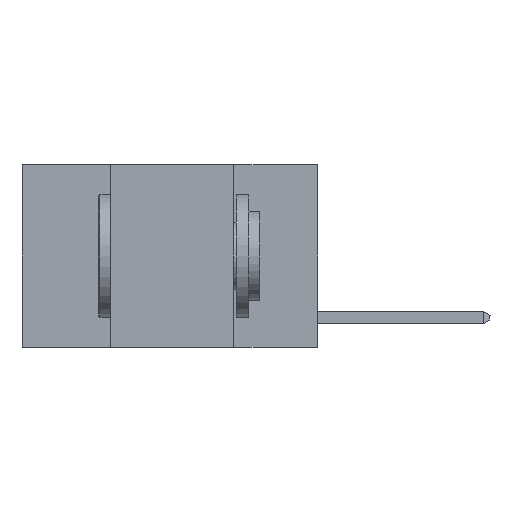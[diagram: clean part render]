
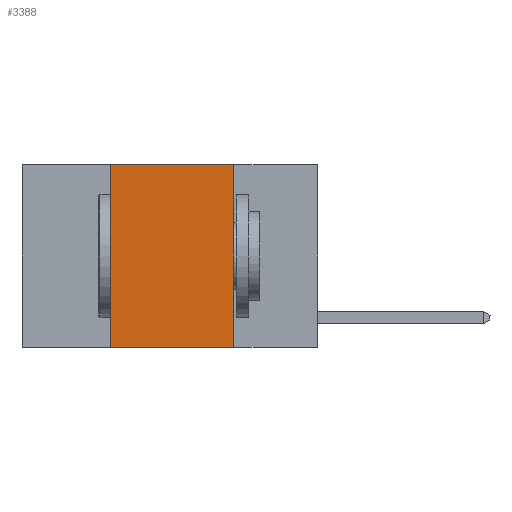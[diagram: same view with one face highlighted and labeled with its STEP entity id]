
A CAD part, left-side view. The second image highlights one B-rep face of the part: STEP entity #3388.
In plain terms, the highlighted planar face has unit normal (-1, 0, 0).
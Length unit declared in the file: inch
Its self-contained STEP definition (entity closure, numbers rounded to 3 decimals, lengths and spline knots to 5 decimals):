
#229 = LINE ( 'NONE', #6430, #9839 ) ;
#306 = CARTESIAN_POINT ( 'NONE',  ( 0., 0.42, -0.37 ) ) ;
#446 = LINE ( 'NONE', #7780, #1799 ) ;
#1441 = AXIS2_PLACEMENT_3D ( 'NONE', #7276, #3364, #8909 ) ;
#1582 = LINE ( 'NONE', #5215, #9831 ) ;
#1799 = VECTOR ( 'NONE', #4607, 39.37008 ) ;
#1932 = CARTESIAN_POINT ( 'NONE',  ( 0., 0.17, -0.37 ) ) ;
#2073 = VERTEX_POINT ( 'NONE', #306 ) ;
#2074 = VERTEX_POINT ( 'NONE', #3468 ) ;
#2099 = ORIENTED_EDGE ( 'NONE', *, *, #2635, .F. ) ;
#2186 = EDGE_CURVE ( 'NONE', #2073, #2074, #229, .T. ) ;
#2592 = PLANE ( 'NONE',  #1441 ) ;
#2635 = EDGE_CURVE ( 'NONE', #2074, #8713, #1582, .T. ) ;
#3364 = DIRECTION ( 'NONE',  ( 1., 0., 0. ) ) ;
#3388 = ADVANCED_FACE ( 'NONE', ( #6554 ), #2592, .F. ) ;
#3468 = CARTESIAN_POINT ( 'NONE',  ( 0., 0.42, 0. ) ) ;
#3784 = VECTOR ( 'NONE', #4148, 39.37008 ) ;
#4148 = DIRECTION ( 'NONE',  ( 0., 0., -1. ) ) ;
#4367 = DIRECTION ( 'NONE',  ( 0., -1., 0. ) ) ;
#4607 = DIRECTION ( 'NONE',  ( 0., -1., 0. ) ) ;
#4779 = EDGE_LOOP ( 'NONE', ( #6652, #2099, #5231, #8162 ) ) ;
#4938 = EDGE_CURVE ( 'NONE', #2073, #9039, #446, .T. ) ;
#5215 = CARTESIAN_POINT ( 'NONE',  ( 0., 0.6, 0. ) ) ;
#5231 = ORIENTED_EDGE ( 'NONE', *, *, #2186, .F. ) ;
#5799 = CARTESIAN_POINT ( 'NONE',  ( 0., 0.17, 0. ) ) ;
#6335 = DIRECTION ( 'NONE',  ( 0., 0., 1. ) ) ;
#6430 = CARTESIAN_POINT ( 'NONE',  ( 0., 0.42, 0. ) ) ;
#6519 = EDGE_CURVE ( 'NONE', #8713, #9039, #7248, .T. ) ;
#6554 = FACE_OUTER_BOUND ( 'NONE', #4779, .T. ) ;
#6652 = ORIENTED_EDGE ( 'NONE', *, *, #6519, .F. ) ;
#7248 = LINE ( 'NONE', #9820, #3784 ) ;
#7276 = CARTESIAN_POINT ( 'NONE',  ( 0., 0.6, 0. ) ) ;
#7780 = CARTESIAN_POINT ( 'NONE',  ( 0., 0.6, -0.37 ) ) ;
#8162 = ORIENTED_EDGE ( 'NONE', *, *, #4938, .T. ) ;
#8713 = VERTEX_POINT ( 'NONE', #5799 ) ;
#8909 = DIRECTION ( 'NONE',  ( 0., 0., -1. ) ) ;
#9039 = VERTEX_POINT ( 'NONE', #1932 ) ;
#9820 = CARTESIAN_POINT ( 'NONE',  ( 0., 0.17, 0. ) ) ;
#9831 = VECTOR ( 'NONE', #4367, 39.37008 ) ;
#9839 = VECTOR ( 'NONE', #6335, 39.37008 ) ;
